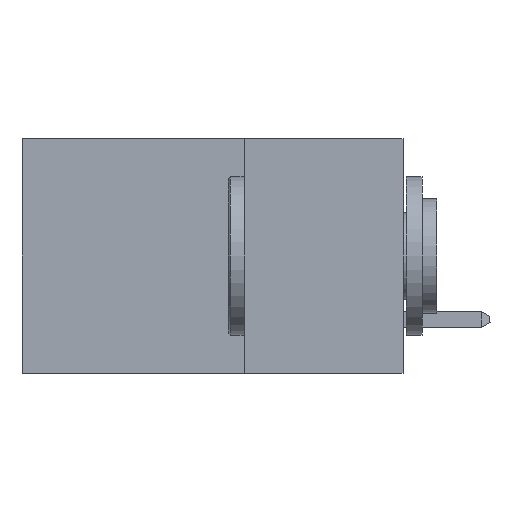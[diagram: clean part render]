
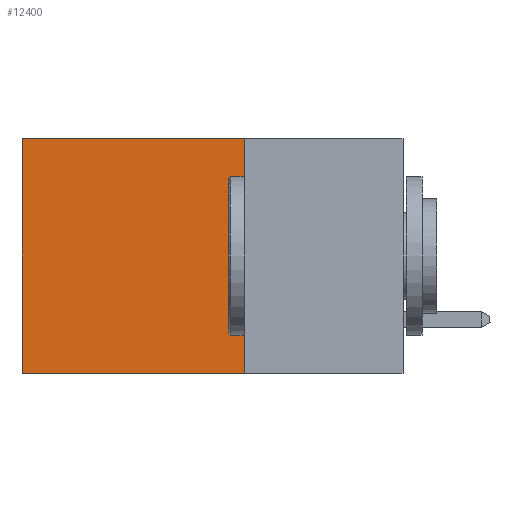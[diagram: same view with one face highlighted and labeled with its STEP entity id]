
A CAD part, left-side view. The second image highlights one B-rep face of the part: STEP entity #12400.
In plain terms, the highlighted planar face has unit normal (-1, 0, 0).
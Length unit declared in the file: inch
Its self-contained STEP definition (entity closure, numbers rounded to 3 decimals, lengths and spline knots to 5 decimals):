
#516 = VERTEX_POINT ( 'NONE', #14667 ) ;
#658 = VECTOR ( 'NONE', #2722, 39.37008 ) ;
#797 = VECTOR ( 'NONE', #6312, 39.37008 ) ;
#1441 = DIRECTION ( 'NONE',  ( 1., 0., 0. ) ) ;
#2088 = VECTOR ( 'NONE', #6554, 39.37008 ) ;
#2663 = EDGE_LOOP ( 'NONE', ( #6654, #17250, #18387, #5448 ) ) ;
#2722 = DIRECTION ( 'NONE',  ( 0., 0., -1. ) ) ;
#2934 = VECTOR ( 'NONE', #11680, 39.37008 ) ;
#3019 = LINE ( 'NONE', #8468, #658 ) ;
#3643 = EDGE_CURVE ( 'NONE', #6060, #18605, #3019, .T. ) ;
#3853 = LINE ( 'NONE', #13678, #797 ) ;
#4453 = LINE ( 'NONE', #10426, #2088 ) ;
#4461 = DIRECTION ( 'NONE',  ( 0., 0., -1. ) ) ;
#5448 = ORIENTED_EDGE ( 'NONE', *, *, #18108, .T. ) ;
#5894 = EDGE_CURVE ( 'NONE', #18605, #516, #3853, .T. ) ;
#6060 = VERTEX_POINT ( 'NONE', #11720 ) ;
#6312 = DIRECTION ( 'NONE',  ( 0., 1., 0. ) ) ;
#6554 = DIRECTION ( 'NONE',  ( 0., 0., -1. ) ) ;
#6654 = ORIENTED_EDGE ( 'NONE', *, *, #15730, .T. ) ;
#7446 = PLANE ( 'NONE',  #15128 ) ;
#8468 = CARTESIAN_POINT ( 'NONE',  ( 0.2875, 0.25, 0. ) ) ;
#10426 = CARTESIAN_POINT ( 'NONE',  ( 0.2875, 0.6, 0. ) ) ;
#11680 = DIRECTION ( 'NONE',  ( 0., 1., 0. ) ) ;
#11720 = CARTESIAN_POINT ( 'NONE',  ( 0.2875, 0.25, 0. ) ) ;
#11792 = LINE ( 'NONE', #18918, #2934 ) ;
#12400 = ADVANCED_FACE ( 'NONE', ( #18797 ), #7446, .F. ) ;
#12468 = VERTEX_POINT ( 'NONE', #13287 ) ;
#13287 = CARTESIAN_POINT ( 'NONE',  ( 0.2875, 0.6, 0. ) ) ;
#13678 = CARTESIAN_POINT ( 'NONE',  ( 0.2875, 0.25, -0.37 ) ) ;
#14667 = CARTESIAN_POINT ( 'NONE',  ( 0.2875, 0.6, -0.37 ) ) ;
#14857 = CARTESIAN_POINT ( 'NONE',  ( 0.2875, 0.25, 0. ) ) ;
#15128 = AXIS2_PLACEMENT_3D ( 'NONE', #14857, #1441, #4461 ) ;
#15730 = EDGE_CURVE ( 'NONE', #12468, #516, #4453, .T. ) ;
#17250 = ORIENTED_EDGE ( 'NONE', *, *, #5894, .F. ) ;
#18108 = EDGE_CURVE ( 'NONE', #6060, #12468, #11792, .T. ) ;
#18387 = ORIENTED_EDGE ( 'NONE', *, *, #3643, .F. ) ;
#18605 = VERTEX_POINT ( 'NONE', #18748 ) ;
#18748 = CARTESIAN_POINT ( 'NONE',  ( 0.2875, 0.25, -0.37 ) ) ;
#18797 = FACE_OUTER_BOUND ( 'NONE', #2663, .T. ) ;
#18918 = CARTESIAN_POINT ( 'NONE',  ( 0.2875, 0.25, 0. ) ) ;
